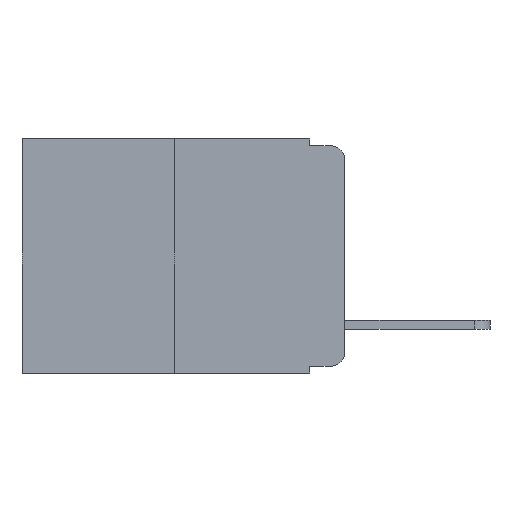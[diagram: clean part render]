
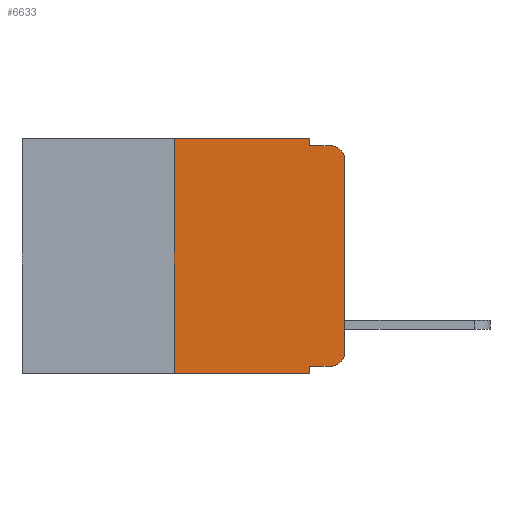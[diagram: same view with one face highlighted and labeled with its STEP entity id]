
A CAD part, left-side view. The second image highlights one B-rep face of the part: STEP entity #6633.
In plain terms, the highlighted planar face has unit normal (-1, 0, 0).
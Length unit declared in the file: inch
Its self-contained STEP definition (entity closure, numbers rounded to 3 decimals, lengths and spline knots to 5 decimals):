
#49 = DIRECTION ( 'NONE',  ( 0., 0., -1. ) ) ;
#224 = CARTESIAN_POINT ( 'NONE',  ( 0., 0.02, -0.01 ) ) ;
#270 = CARTESIAN_POINT ( 'NONE',  ( 0., 0.051, -0.343 ) ) ;
#274 = CIRCLE ( 'NONE', #1974, 0.02 ) ;
#487 = CIRCLE ( 'NONE', #3826, 0.02 ) ;
#532 = CARTESIAN_POINT ( 'NONE',  ( 0., 0.25, 0. ) ) ;
#664 = DIRECTION ( 'NONE',  ( -1., 0., 0. ) ) ;
#799 = LINE ( 'NONE', #4275, #8545 ) ;
#995 = VECTOR ( 'NONE', #4186, 39.37008 ) ;
#1179 = VERTEX_POINT ( 'NONE', #4307 ) ;
#1181 = EDGE_LOOP ( 'NONE', ( #9754, #9409, #5952, #6426, #5661, #5790, #3425, #8132, #10993, #5384 ) ) ;
#1204 = LINE ( 'NONE', #532, #11166 ) ;
#1406 = VERTEX_POINT ( 'NONE', #224 ) ;
#1430 = EDGE_CURVE ( 'NONE', #9317, #5155, #487, .T. ) ;
#1461 = CARTESIAN_POINT ( 'NONE',  ( 0., 0.051, -0.01 ) ) ;
#1489 = EDGE_CURVE ( 'NONE', #8652, #3828, #4225, .T. ) ;
#1956 = FACE_OUTER_BOUND ( 'NONE', #1181, .T. ) ;
#1970 = EDGE_CURVE ( 'NONE', #10598, #2919, #3647, .T. ) ;
#1974 = AXIS2_PLACEMENT_3D ( 'NONE', #2652, #10631, #5375 ) ;
#2362 = VERTEX_POINT ( 'NONE', #2479 ) ;
#2479 = CARTESIAN_POINT ( 'NONE',  ( 0., 0., -0.03 ) ) ;
#2652 = CARTESIAN_POINT ( 'NONE',  ( 0., 0.02, -0.03 ) ) ;
#2690 = CARTESIAN_POINT ( 'NONE',  ( 0., 0.473, 0. ) ) ;
#2919 = VERTEX_POINT ( 'NONE', #8678 ) ;
#3047 = LINE ( 'NONE', #1461, #995 ) ;
#3145 = LINE ( 'NONE', #9289, #7590 ) ;
#3224 = EDGE_CURVE ( 'NONE', #8652, #10598, #1204, .T. ) ;
#3425 = ORIENTED_EDGE ( 'NONE', *, *, #1489, .T. ) ;
#3647 = LINE ( 'NONE', #2690, #7805 ) ;
#3826 = AXIS2_PLACEMENT_3D ( 'NONE', #8759, #664, #6094 ) ;
#3828 = VERTEX_POINT ( 'NONE', #270 ) ;
#4186 = DIRECTION ( 'NONE',  ( 0., -1., 0. ) ) ;
#4225 = LINE ( 'NONE', #4928, #5779 ) ;
#4275 = CARTESIAN_POINT ( 'NONE',  ( 0., 0.051, -0.333 ) ) ;
#4305 = DIRECTION ( 'NONE',  ( 1., 0., 0. ) ) ;
#4307 = CARTESIAN_POINT ( 'NONE',  ( 0., 0.051, -0.333 ) ) ;
#4392 = CARTESIAN_POINT ( 'NONE',  ( 0., 0.25, -0.343 ) ) ;
#4928 = CARTESIAN_POINT ( 'NONE',  ( 0., 0.473, -0.343 ) ) ;
#5155 = VERTEX_POINT ( 'NONE', #9801 ) ;
#5356 = DIRECTION ( 'NONE',  ( 0., -1., 0. ) ) ;
#5375 = DIRECTION ( 'NONE',  ( 0., 0., -1. ) ) ;
#5384 = ORIENTED_EDGE ( 'NONE', *, *, #1430, .T. ) ;
#5422 = DIRECTION ( 'NONE',  ( 0., 0., -1. ) ) ;
#5661 = ORIENTED_EDGE ( 'NONE', *, *, #1970, .F. ) ;
#5779 = VECTOR ( 'NONE', #8593, 39.37008 ) ;
#5790 = ORIENTED_EDGE ( 'NONE', *, *, #3224, .F. ) ;
#5797 = CARTESIAN_POINT ( 'NONE',  ( 0., 0.25, 0. ) ) ;
#5926 = CARTESIAN_POINT ( 'NONE',  ( 0., 0.051, -0.01 ) ) ;
#5952 = ORIENTED_EDGE ( 'NONE', *, *, #6576, .F. ) ;
#6094 = DIRECTION ( 'NONE',  ( 0., 0., -1. ) ) ;
#6170 = EDGE_CURVE ( 'NONE', #1179, #9317, #799, .T. ) ;
#6426 = ORIENTED_EDGE ( 'NONE', *, *, #8873, .F. ) ;
#6576 = EDGE_CURVE ( 'NONE', #10021, #1406, #3047, .T. ) ;
#6633 = ADVANCED_FACE ( 'NONE', ( #1956 ), #6945, .F. ) ;
#6692 = CARTESIAN_POINT ( 'NONE',  ( 0., 0.02, -0.333 ) ) ;
#6713 = DIRECTION ( 'NONE',  ( 0., 0., 1. ) ) ;
#6945 = PLANE ( 'NONE',  #11227 ) ;
#7172 = DIRECTION ( 'NONE',  ( 0., -1., 0. ) ) ;
#7590 = VECTOR ( 'NONE', #6713, 39.37008 ) ;
#7805 = VECTOR ( 'NONE', #7172, 39.37008 ) ;
#7895 = CARTESIAN_POINT ( 'NONE',  ( 0., 0.051, 0. ) ) ;
#8132 = ORIENTED_EDGE ( 'NONE', *, *, #10915, .F. ) ;
#8151 = LINE ( 'NONE', #8734, #10886 ) ;
#8301 = VECTOR ( 'NONE', #5422, 39.37008 ) ;
#8545 = VECTOR ( 'NONE', #5356, 39.37008 ) ;
#8593 = DIRECTION ( 'NONE',  ( 0., -1., 0. ) ) ;
#8652 = VERTEX_POINT ( 'NONE', #4392 ) ;
#8678 = CARTESIAN_POINT ( 'NONE',  ( 0., 0.051, 0. ) ) ;
#8710 = LINE ( 'NONE', #7895, #8301 ) ;
#8734 = CARTESIAN_POINT ( 'NONE',  ( 0., 0.051, 0. ) ) ;
#8759 = CARTESIAN_POINT ( 'NONE',  ( 0., 0.02, -0.313 ) ) ;
#8873 = EDGE_CURVE ( 'NONE', #2919, #10021, #8710, .T. ) ;
#9007 = EDGE_CURVE ( 'NONE', #2362, #1406, #274, .T. ) ;
#9090 = DIRECTION ( 'NONE',  ( 0., 0., -1. ) ) ;
#9245 = DIRECTION ( 'NONE',  ( 0., 0., 1. ) ) ;
#9289 = CARTESIAN_POINT ( 'NONE',  ( 0., 0., 0. ) ) ;
#9317 = VERTEX_POINT ( 'NONE', #6692 ) ;
#9409 = ORIENTED_EDGE ( 'NONE', *, *, #9007, .T. ) ;
#9752 = CARTESIAN_POINT ( 'NONE',  ( 0., 0.473, 0. ) ) ;
#9754 = ORIENTED_EDGE ( 'NONE', *, *, #9965, .T. ) ;
#9801 = CARTESIAN_POINT ( 'NONE',  ( 0., 0., -0.313 ) ) ;
#9965 = EDGE_CURVE ( 'NONE', #5155, #2362, #3145, .T. ) ;
#10021 = VERTEX_POINT ( 'NONE', #5926 ) ;
#10598 = VERTEX_POINT ( 'NONE', #5797 ) ;
#10631 = DIRECTION ( 'NONE',  ( -1., 0., 0. ) ) ;
#10886 = VECTOR ( 'NONE', #9090, 39.37008 ) ;
#10915 = EDGE_CURVE ( 'NONE', #1179, #3828, #8151, .T. ) ;
#10993 = ORIENTED_EDGE ( 'NONE', *, *, #6170, .T. ) ;
#11166 = VECTOR ( 'NONE', #9245, 39.37008 ) ;
#11227 = AXIS2_PLACEMENT_3D ( 'NONE', #9752, #4305, #49 ) ;
